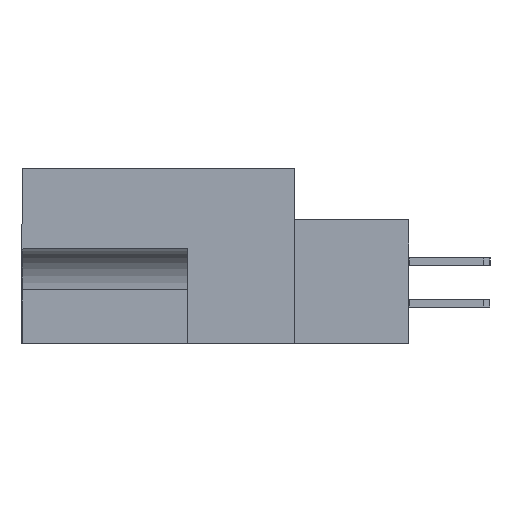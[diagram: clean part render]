
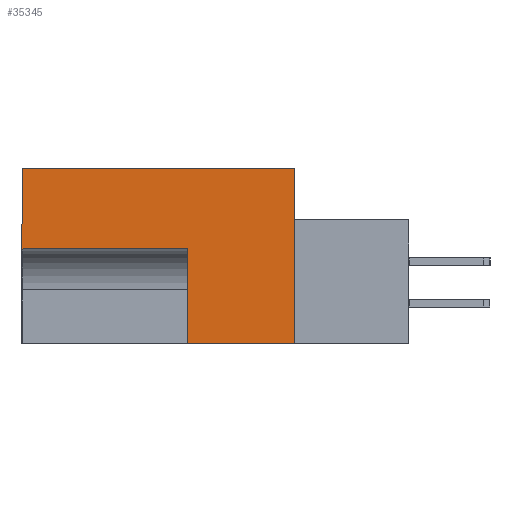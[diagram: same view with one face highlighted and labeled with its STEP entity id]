
A CAD part, left-side view. The second image highlights one B-rep face of the part: STEP entity #35345.
In plain terms, the highlighted planar face has unit normal (-1, 0, 0).
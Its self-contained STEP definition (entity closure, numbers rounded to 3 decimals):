
#868 = LINE ( 'NONE', #32211, #35476 ) ;
#2228 = CARTESIAN_POINT ( 'NONE',  ( 0., 0., 0. ) ) ;
#2415 = VECTOR ( 'NONE', #26134, 1000. ) ;
#3871 = CARTESIAN_POINT ( 'NONE',  ( 0., 11.506, 0. ) ) ;
#3908 = LINE ( 'NONE', #3871, #2415 ) ;
#4369 = EDGE_LOOP ( 'NONE', ( #22889, #27786, #13140, #12005, #22110, #37397 ) ) ;
#5100 = DIRECTION ( 'NONE',  ( 0., 0., 1. ) ) ;
#5364 = EDGE_CURVE ( 'NONE', #39493, #9127, #3908, .T. ) ;
#5399 = VERTEX_POINT ( 'NONE', #29450 ) ;
#6229 = CARTESIAN_POINT ( 'NONE',  ( 0., 0., 0. ) ) ;
#6747 = EDGE_CURVE ( 'NONE', #9127, #39070, #6780, .T. ) ;
#6780 = LINE ( 'NONE', #6229, #38397 ) ;
#9009 = CARTESIAN_POINT ( 'NONE',  ( 0., 0., 0. ) ) ;
#9127 = VERTEX_POINT ( 'NONE', #2228 ) ;
#12005 = ORIENTED_EDGE ( 'NONE', *, *, #24022, .F. ) ;
#12436 = VECTOR ( 'NONE', #40027, 1000. ) ;
#12725 = LINE ( 'NONE', #24194, #40392 ) ;
#13140 = ORIENTED_EDGE ( 'NONE', *, *, #5364, .F. ) ;
#13283 = DIRECTION ( 'NONE',  ( 0., 1., 0. ) ) ;
#15025 = CARTESIAN_POINT ( 'NONE',  ( 0., -8.814, -13.487 ) ) ;
#15206 = PLANE ( 'NONE',  #26147 ) ;
#15220 = VERTEX_POINT ( 'NONE', #33207 ) ;
#17217 = VERTEX_POINT ( 'NONE', #22583 ) ;
#17226 = EDGE_CURVE ( 'NONE', #5399, #15220, #868, .T. ) ;
#18885 = DIRECTION ( 'NONE',  ( 0., 0., 1. ) ) ;
#21475 = EDGE_CURVE ( 'NONE', #17217, #5399, #33212, .T. ) ;
#21853 = DIRECTION ( 'NONE',  ( 0., 0., -1. ) ) ;
#22110 = ORIENTED_EDGE ( 'NONE', *, *, #17226, .F. ) ;
#22583 = CARTESIAN_POINT ( 'NONE',  ( 0., 8.255, -13.487 ) ) ;
#22889 = ORIENTED_EDGE ( 'NONE', *, *, #40244, .F. ) ;
#23854 = FACE_OUTER_BOUND ( 'NONE', #4369, .T. ) ;
#24022 = EDGE_CURVE ( 'NONE', #15220, #39493, #12725, .T. ) ;
#24194 = CARTESIAN_POINT ( 'NONE',  ( 0., 20.955, -13.487 ) ) ;
#24353 = VECTOR ( 'NONE', #18885, 1000. ) ;
#25168 = DIRECTION ( 'NONE',  ( 0., 0., -1. ) ) ;
#26018 = CARTESIAN_POINT ( 'NONE',  ( 0., 20.955, 0. ) ) ;
#26134 = DIRECTION ( 'NONE',  ( 0., -1., 0. ) ) ;
#26147 = AXIS2_PLACEMENT_3D ( 'NONE', #9009, #37713, #21853 ) ;
#26812 = LINE ( 'NONE', #15025, #12436 ) ;
#27786 = ORIENTED_EDGE ( 'NONE', *, *, #6747, .F. ) ;
#29450 = CARTESIAN_POINT ( 'NONE',  ( 0., 8.255, -6.172 ) ) ;
#31443 = CARTESIAN_POINT ( 'NONE',  ( 0., 8.255, -13.487 ) ) ;
#32211 = CARTESIAN_POINT ( 'NONE',  ( 0., 8.255, -6.172 ) ) ;
#33207 = CARTESIAN_POINT ( 'NONE',  ( 0., 20.955, -6.172 ) ) ;
#33212 = LINE ( 'NONE', #31443, #24353 ) ;
#35345 = ADVANCED_FACE ( 'NONE', ( #23854 ), #15206, .F. ) ;
#35476 = VECTOR ( 'NONE', #13283, 1000. ) ;
#36813 = CARTESIAN_POINT ( 'NONE',  ( 0., 0., -13.487 ) ) ;
#37397 = ORIENTED_EDGE ( 'NONE', *, *, #21475, .F. ) ;
#37713 = DIRECTION ( 'NONE',  ( 1., 0., 0. ) ) ;
#38397 = VECTOR ( 'NONE', #25168, 1000. ) ;
#39070 = VERTEX_POINT ( 'NONE', #36813 ) ;
#39493 = VERTEX_POINT ( 'NONE', #26018 ) ;
#40027 = DIRECTION ( 'NONE',  ( 0., 1., 0. ) ) ;
#40244 = EDGE_CURVE ( 'NONE', #39070, #17217, #26812, .T. ) ;
#40392 = VECTOR ( 'NONE', #5100, 1000. ) ;
